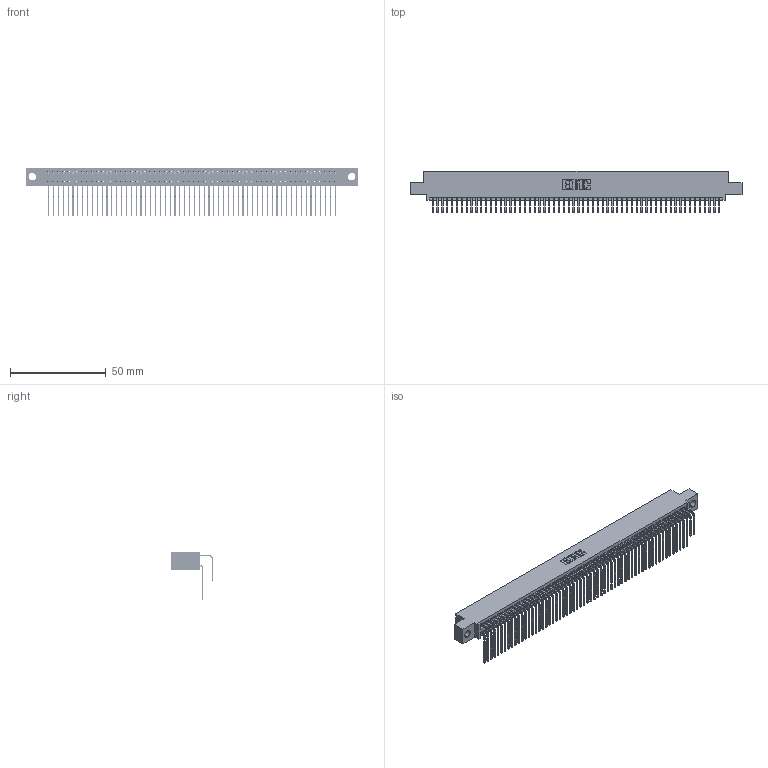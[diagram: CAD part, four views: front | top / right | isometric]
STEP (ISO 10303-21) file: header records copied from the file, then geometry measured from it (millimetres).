
FILE_DESCRIPTION (( 'STEP AP203' ), '1' );
FILE_NAME ('345-120-558-504.STEP', '2021-05-25T17:12:41', ( '' ), ( '' ), 'SwSTEP 2.0', 'SolidWorks 2020', '' );
FILE_SCHEMA (( 'CONFIG_CONTROL_DESIGN' ));
Length unit declared in the file: inch
Products named in the file (4): 345-120-558-504; 345-292-001_558 Tail - 2; 345-292-001_558 559 Tail - 1; 345 Part_0.110 Offset - 0.156 Dia-TI
Assembly tree (121 placements, depth 2):
  345-120-558-504
    345 Part_0.110 Offset - 0.156 Dia-TI
    345-292-001_558 559 Tail - 1  x60
    345-292-001_558 Tail - 2  x60
Bounding box: 173.61 x 21.83 x 25.53 mm (x, y, z)
Volume: 17544.6 mm3; surface area: 29482.1 mm2
Topology: 121 solids, 121 shells, 6384 faces, 18989 edges, 12498 vertices
Faces by surface type: plane 4298, cylinder 2086
Entity records: 46857 total; most frequent: CARTESIAN_POINT 7889, ORIENTED_EDGE 7770, DIRECTION 6905, EDGE_CURVE 3885, VECTOR 3473, LINE 3473, VERTEX_POINT 2586, AXIS2_PLACEMENT_3D 1716
